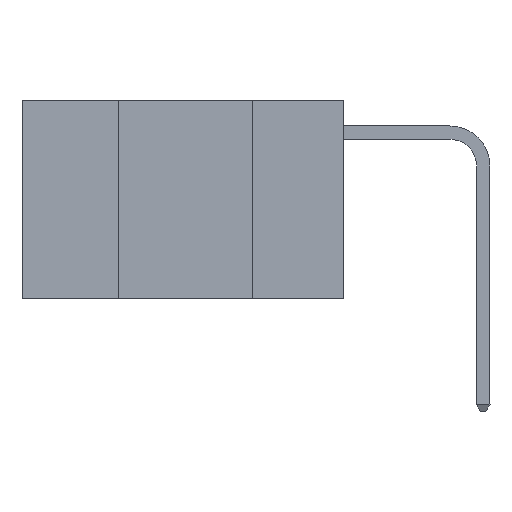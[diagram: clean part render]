
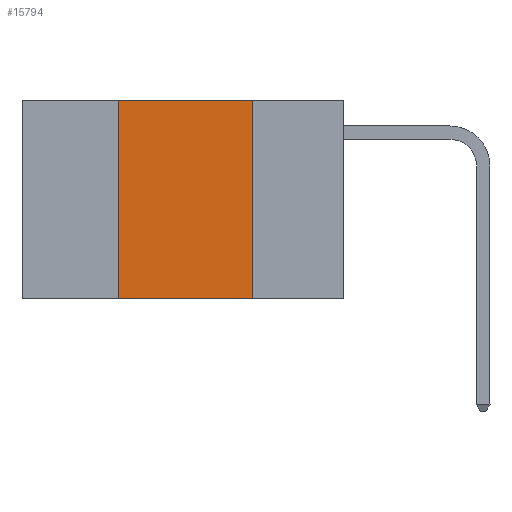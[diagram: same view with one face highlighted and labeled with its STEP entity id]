
A CAD part, left-side view. The second image highlights one B-rep face of the part: STEP entity #15794.
In plain terms, the highlighted planar face has unit normal (-1, 0, 0).
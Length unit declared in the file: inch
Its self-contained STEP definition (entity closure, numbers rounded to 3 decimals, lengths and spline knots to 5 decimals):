
#742 = CARTESIAN_POINT ( 'NONE',  ( 0., 0.17, 0. ) ) ;
#990 = DIRECTION ( 'NONE',  ( 0., 0., -1. ) ) ;
#3147 = VECTOR ( 'NONE', #990, 39.37008 ) ;
#3736 = PLANE ( 'NONE',  #14094 ) ;
#3760 = VECTOR ( 'NONE', #12179, 39.37008 ) ;
#3840 = DIRECTION ( 'NONE',  ( 0., 0., 1. ) ) ;
#4181 = DIRECTION ( 'NONE',  ( 0., -1., 0. ) ) ;
#4208 = EDGE_CURVE ( 'NONE', #16232, #11408, #5259, .T. ) ;
#4840 = ORIENTED_EDGE ( 'NONE', *, *, #6032, .F. ) ;
#5259 = LINE ( 'NONE', #13593, #3147 ) ;
#6032 = EDGE_CURVE ( 'NONE', #10148, #16232, #9626, .T. ) ;
#6388 = CARTESIAN_POINT ( 'NONE',  ( 0., 0.6, 0. ) ) ;
#6655 = CARTESIAN_POINT ( 'NONE',  ( 0., 0.6, 0. ) ) ;
#6985 = LINE ( 'NONE', #12418, #16026 ) ;
#7207 = EDGE_CURVE ( 'NONE', #11914, #10148, #8044, .T. ) ;
#7698 = EDGE_CURVE ( 'NONE', #11914, #11408, #6985, .T. ) ;
#7857 = VECTOR ( 'NONE', #3840, 39.37008 ) ;
#8044 = LINE ( 'NONE', #12203, #7857 ) ;
#9626 = LINE ( 'NONE', #6655, #3760 ) ;
#9975 = ORIENTED_EDGE ( 'NONE', *, *, #4208, .F. ) ;
#10148 = VERTEX_POINT ( 'NONE', #14863 ) ;
#11408 = VERTEX_POINT ( 'NONE', #13313 ) ;
#11753 = ORIENTED_EDGE ( 'NONE', *, *, #7698, .T. ) ;
#11914 = VERTEX_POINT ( 'NONE', #15397 ) ;
#12179 = DIRECTION ( 'NONE',  ( 0., -1., 0. ) ) ;
#12203 = CARTESIAN_POINT ( 'NONE',  ( 0., 0.42, 0. ) ) ;
#12418 = CARTESIAN_POINT ( 'NONE',  ( 0., 0.6, -0.37 ) ) ;
#13313 = CARTESIAN_POINT ( 'NONE',  ( 0., 0.17, -0.37 ) ) ;
#13461 = FACE_OUTER_BOUND ( 'NONE', #14834, .T. ) ;
#13593 = CARTESIAN_POINT ( 'NONE',  ( 0., 0.17, 0. ) ) ;
#14094 = AXIS2_PLACEMENT_3D ( 'NONE', #6388, #17482, #17390 ) ;
#14834 = EDGE_LOOP ( 'NONE', ( #9975, #4840, #17196, #11753 ) ) ;
#14863 = CARTESIAN_POINT ( 'NONE',  ( 0., 0.42, 0. ) ) ;
#15397 = CARTESIAN_POINT ( 'NONE',  ( 0., 0.42, -0.37 ) ) ;
#15794 = ADVANCED_FACE ( 'NONE', ( #13461 ), #3736, .F. ) ;
#16026 = VECTOR ( 'NONE', #4181, 39.37008 ) ;
#16232 = VERTEX_POINT ( 'NONE', #742 ) ;
#17196 = ORIENTED_EDGE ( 'NONE', *, *, #7207, .F. ) ;
#17390 = DIRECTION ( 'NONE',  ( 0., 0., -1. ) ) ;
#17482 = DIRECTION ( 'NONE',  ( 1., 0., 0. ) ) ;
